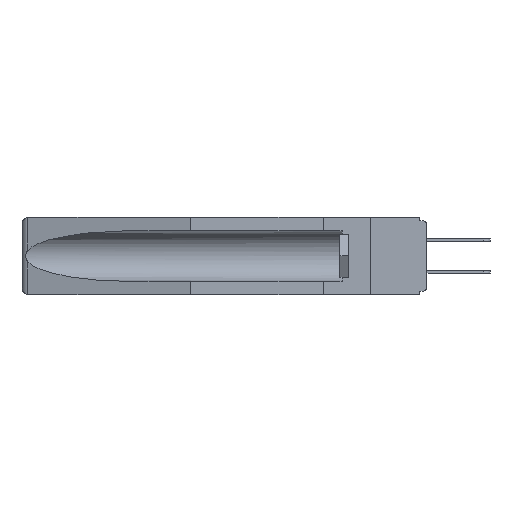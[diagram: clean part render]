
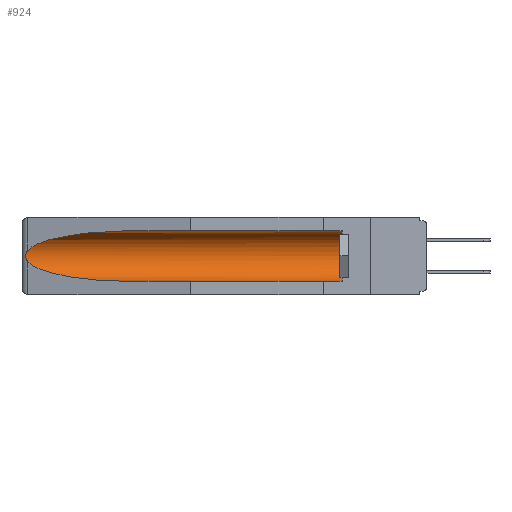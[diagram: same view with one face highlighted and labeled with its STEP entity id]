
A CAD part, left-side view. The second image highlights one B-rep face of the part: STEP entity #924.
In plain terms, the highlighted cylindrical face has radius 2.857 mm (diameter 5.715 mm), a partial arc.
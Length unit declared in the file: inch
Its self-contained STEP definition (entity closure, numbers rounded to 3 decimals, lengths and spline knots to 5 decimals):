
#131 = EDGE_CURVE ( 'NONE', #19028, #8671, #2958, .T. ) ;
#853 = AXIS2_PLACEMENT_3D ( 'NONE', #20297, #22253, #4865 ) ;
#924 = ADVANCED_FACE ( 'NONE', ( #12405 ), #989, .F. ) ;
#989 = CYLINDRICAL_SURFACE ( 'NONE', #10025, 0.1125 ) ;
#1293 = EDGE_CURVE ( 'NONE', #19028, #22481, #22903, .T. ) ;
#1345 = VERTEX_POINT ( 'NONE', #22058 ) ;
#1854 = CARTESIAN_POINT ( 'NONE',  ( 0.2675, 1.53308, -0.17534 ) ) ;
#2004 = CARTESIAN_POINT ( 'NONE',  ( 0.155, -0.30754, -0.1715 ) ) ;
#2110 = CARTESIAN_POINT ( 'NONE',  ( 0.2673, 1.53269, -0.17917 ) ) ;
#2178 = CARTESIAN_POINT ( 'NONE',  ( 0.21114, 1.30732, -0.284 ) ) ;
#2619 = CARTESIAN_POINT ( 'NONE',  ( 0.25451, 1.48313, -0.09465 ) ) ;
#2647 =( BOUNDED_CURVE ( )  B_SPLINE_CURVE ( 3, ( #8210, #15941, #2619, #16017 ),
 .UNSPECIFIED., .F., .F. ) 
 B_SPLINE_CURVE_WITH_KNOTS ( ( 4, 4 ),
 ( 4.71239, 6.08839 ),
 .UNSPECIFIED. ) 
 CURVE ( )  GEOMETRIC_REPRESENTATION_ITEM ( )  RATIONAL_B_SPLINE_CURVE ( ( 1., 0.848, 0.848, 1. ) ) 
 REPRESENTATION_ITEM ( '' )  );
#2958 = CIRCLE ( 'NONE', #853, 0.1125 ) ;
#3160 = CARTESIAN_POINT ( 'NONE',  ( 0.26537, 1.52718, -0.14972 ) ) ;
#3445 = ORIENTED_EDGE ( 'NONE', *, *, #131, .T. ) ;
#3522 = ORIENTED_EDGE ( 'NONE', *, *, #10136, .T. ) ;
#3762 = CARTESIAN_POINT ( 'NONE',  ( 0.26655, 1.53094, -0.18657 ) ) ;
#4865 = DIRECTION ( 'NONE',  ( 0., 0., 1. ) ) ;
#5005 = CARTESIAN_POINT ( 'NONE',  ( 0.26537, 1.52718, -0.19328 ) ) ;
#5382 = VERTEX_POINT ( 'NONE', #3160 ) ;
#6030 = CARTESIAN_POINT ( 'NONE',  ( 0.155, 1.07973, -0.284 ) ) ;
#6460 = ORIENTED_EDGE ( 'NONE', *, *, #14481, .T. ) ;
#8210 = CARTESIAN_POINT ( 'NONE',  ( 0.155, 1.07973, -0.059 ) ) ;
#8419 =( BOUNDED_CURVE ( )  B_SPLINE_CURVE ( 3, ( #10108, #12057, #2178, #6030 ),
 .UNSPECIFIED., .F., .F. ) 
 B_SPLINE_CURVE_WITH_KNOTS ( ( 4, 4 ),
 ( 0.1948, 1.5708 ),
 .UNSPECIFIED. ) 
 CURVE ( )  GEOMETRIC_REPRESENTATION_ITEM ( )  RATIONAL_B_SPLINE_CURVE ( ( 1., 0.848, 0.848, 1. ) ) 
 REPRESENTATION_ITEM ( '' )  );
#8671 = VERTEX_POINT ( 'NONE', #12744 ) ;
#8778 = CARTESIAN_POINT ( 'NONE',  ( 0.155, 0.126, -0.284 ) ) ;
#9841 = DIRECTION ( 'NONE',  ( 0., 0., 1. ) ) ;
#10025 = AXIS2_PLACEMENT_3D ( 'NONE', #2004, #11716, #9841 ) ;
#10108 = CARTESIAN_POINT ( 'NONE',  ( 0.26537, 1.52718, -0.19328 ) ) ;
#10136 = EDGE_CURVE ( 'NONE', #5382, #21296, #22357, .T. ) ;
#10629 = CARTESIAN_POINT ( 'NONE',  ( 0.26537, 1.52718, -0.19328 ) ) ;
#11716 = DIRECTION ( 'NONE',  ( 0., 1., 0. ) ) ;
#12057 = CARTESIAN_POINT ( 'NONE',  ( 0.25451, 1.48313, -0.24835 ) ) ;
#12405 = FACE_OUTER_BOUND ( 'NONE', #24623, .T. ) ;
#12485 = CARTESIAN_POINT ( 'NONE',  ( 0.155, -0.30754, -0.059 ) ) ;
#12744 = CARTESIAN_POINT ( 'NONE',  ( 0.155, 0.126, -0.059 ) ) ;
#12942 = VECTOR ( 'NONE', #23994, 39.37008 ) ;
#13162 = ORIENTED_EDGE ( 'NONE', *, *, #23148, .T. ) ;
#14481 = EDGE_CURVE ( 'NONE', #1345, #5382, #2647, .T. ) ;
#15941 = CARTESIAN_POINT ( 'NONE',  ( 0.21114, 1.30732, -0.059 ) ) ;
#15991 = ORIENTED_EDGE ( 'NONE', *, *, #18277, .T. ) ;
#16017 = CARTESIAN_POINT ( 'NONE',  ( 0.26537, 1.52718, -0.14972 ) ) ;
#17200 = CARTESIAN_POINT ( 'NONE',  ( 0.26597, 1.5296, -0.19026 ) ) ;
#17364 = CARTESIAN_POINT ( 'NONE',  ( 0.155, 1.07973, -0.284 ) ) ;
#17375 = CARTESIAN_POINT ( 'NONE',  ( 0.26597, 1.52961, -0.15275 ) ) ;
#18081 = DIRECTION ( 'NONE',  ( 0., 1., 0. ) ) ;
#18277 = EDGE_CURVE ( 'NONE', #21296, #22481, #8419, .T. ) ;
#19028 = VERTEX_POINT ( 'NONE', #8778 ) ;
#19281 = CARTESIAN_POINT ( 'NONE',  ( 0.2673, 1.5327, -0.16383 ) ) ;
#19365 = CARTESIAN_POINT ( 'NONE',  ( 0.26537, 1.52718, -0.14972 ) ) ;
#19590 = VECTOR ( 'NONE', #18081, 39.37008 ) ;
#20281 = CARTESIAN_POINT ( 'NONE',  ( 0.155, -0.30754, -0.284 ) ) ;
#20297 = CARTESIAN_POINT ( 'NONE',  ( 0.155, 0.126, -0.1715 ) ) ;
#21296 = VERTEX_POINT ( 'NONE', #5005 ) ;
#22058 = CARTESIAN_POINT ( 'NONE',  ( 0.155, 1.07973, -0.059 ) ) ;
#22253 = DIRECTION ( 'NONE',  ( 0., -1., 0. ) ) ;
#22357 = B_SPLINE_CURVE_WITH_KNOTS ( 'NONE', 3,
 ( #19365, #17375, #24762, #19281, #24856, #1854, #2110, #3762, #17200, #10629 ),
 .UNSPECIFIED., .F., .F.,
 ( 4, 2, 2, 2, 4 ),
 ( 0., 0.00029, 0.00058, 0.00087, 0.00117 ),
 .UNSPECIFIED. ) ;
#22481 = VERTEX_POINT ( 'NONE', #17364 ) ;
#22903 = LINE ( 'NONE', #20281, #12942 ) ;
#23148 = EDGE_CURVE ( 'NONE', #8671, #1345, #24703, .T. ) ;
#23376 = ORIENTED_EDGE ( 'NONE', *, *, #1293, .F. ) ;
#23994 = DIRECTION ( 'NONE',  ( 0., 1., 0. ) ) ;
#24623 = EDGE_LOOP ( 'NONE', ( #6460, #3522, #15991, #23376, #3445, #13162 ) ) ;
#24703 = LINE ( 'NONE', #12485, #19590 ) ;
#24762 = CARTESIAN_POINT ( 'NONE',  ( 0.26654, 1.53092, -0.15636 ) ) ;
#24856 = CARTESIAN_POINT ( 'NONE',  ( 0.2675, 1.53308, -0.16763 ) ) ;
